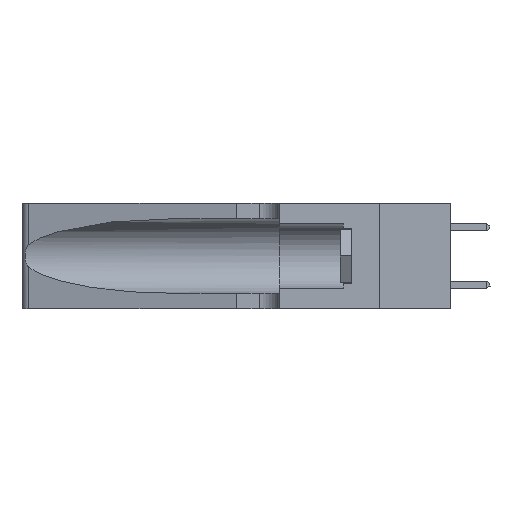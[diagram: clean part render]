
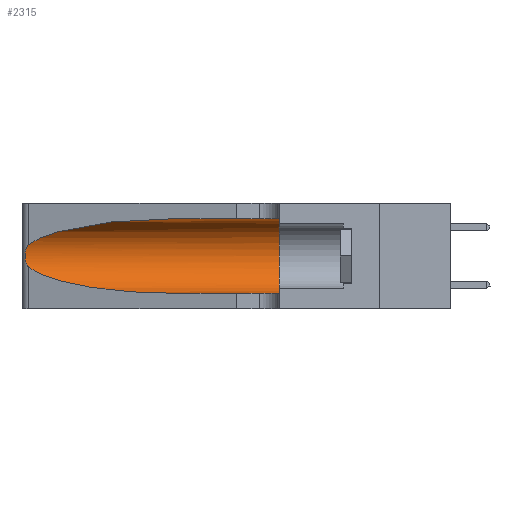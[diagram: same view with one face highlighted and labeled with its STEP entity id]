
A CAD part, left-side view. The second image highlights one B-rep face of the part: STEP entity #2315.
In plain terms, the highlighted cylindrical face has radius 3.308 mm (diameter 6.617 mm), a partial arc.
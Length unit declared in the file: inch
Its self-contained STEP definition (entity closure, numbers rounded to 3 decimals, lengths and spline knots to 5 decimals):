
#126 = CARTESIAN_POINT ( 'NONE',  ( 0.26018, 1.23835, 0.19895 ) ) ;
#447 = EDGE_CURVE ( 'NONE', #9253, #2792, #9507, .T. ) ;
#688 = CARTESIAN_POINT ( 'NONE',  ( 0.25487, 1.22718, 0.22369 ) ) ;
#937 =( BOUNDED_CURVE ( )  B_SPLINE_CURVE ( 3, ( #8725, #13086, #7332, #17427 ),
 .UNSPECIFIED., .F., .T. ) 
 B_SPLINE_CURVE_WITH_KNOTS ( ( 4, 4 ),
 ( 3.44316, 4.71239 ),
 .UNSPECIFIED. ) 
 CURVE ( )  GEOMETRIC_REPRESENTATION_ITEM ( )  RATIONAL_B_SPLINE_CURVE ( ( 1., 0.87, 0.87, 1. ) ) 
 REPRESENTATION_ITEM ( '' )  );
#1132 = EDGE_CURVE ( 'NONE', #12145, #8710, #11768, .T. ) ;
#1556 = DIRECTION ( 'NONE',  ( 0., -1., 0. ) ) ;
#1603 = CARTESIAN_POINT ( 'NONE',  ( 0.26075, 1.23896, 0.178 ) ) ;
#2315 = ADVANCED_FACE ( 'NONE', ( #3264 ), #13948, .F. ) ;
#2553 = VECTOR ( 'NONE', #12333, 39.37008 ) ;
#2683 = AXIS2_PLACEMENT_3D ( 'NONE', #3656, #12179, #5624 ) ;
#2792 = VERTEX_POINT ( 'NONE', #5924 ) ;
#3127 = CARTESIAN_POINT ( 'NONE',  ( 0.25856, 1.23593, 0.16098 ) ) ;
#3264 = FACE_OUTER_BOUND ( 'NONE', #5258, .T. ) ;
#3307 = EDGE_CURVE ( 'NONE', #7246, #2792, #6495, .T. ) ;
#3656 = CARTESIAN_POINT ( 'NONE',  ( 0.1305, 0.35, 0.185 ) ) ;
#4102 = ORIENTED_EDGE ( 'NONE', *, *, #3307, .T. ) ;
#4619 = CARTESIAN_POINT ( 'NONE',  ( 0.25639, 1.23186, 0.15144 ) ) ;
#4813 = DIRECTION ( 'NONE',  ( 0., -1., 0. ) ) ;
#5023 = CARTESIAN_POINT ( 'NONE',  ( 0.1305, 0.35, 0.31525 ) ) ;
#5258 = EDGE_LOOP ( 'NONE', ( #7559, #9914, #7156, #4102, #18725, #17137 ) ) ;
#5624 = DIRECTION ( 'NONE',  ( 0., 0., 1. ) ) ;
#5688 = AXIS2_PLACEMENT_3D ( 'NONE', #9655, #4813, #15910 ) ;
#5924 = CARTESIAN_POINT ( 'NONE',  ( 0.1305, 0.35, 0.05475 ) ) ;
#6111 = CARTESIAN_POINT ( 'NONE',  ( 0.25487, 1.22718, 0.14631 ) ) ;
#6495 = LINE ( 'NONE', #6636, #2553 ) ;
#6636 = CARTESIAN_POINT ( 'NONE',  ( 0.1305, 1.61858, 0.05475 ) ) ;
#6849 = VERTEX_POINT ( 'NONE', #12609 ) ;
#7074 = EDGE_CURVE ( 'NONE', #6849, #7246, #937, .T. ) ;
#7111 = CARTESIAN_POINT ( 'NONE',  ( 0.1305, 0.72297, 0.31525 ) ) ;
#7156 = ORIENTED_EDGE ( 'NONE', *, *, #7074, .T. ) ;
#7246 = VERTEX_POINT ( 'NONE', #10557 ) ;
#7332 = CARTESIAN_POINT ( 'NONE',  ( 0.18966, 0.96281, 0.05475 ) ) ;
#7487 = CARTESIAN_POINT ( 'NONE',  ( 0.25639, 1.23184, 0.21858 ) ) ;
#7559 = ORIENTED_EDGE ( 'NONE', *, *, #1132, .T. ) ;
#8710 = VERTEX_POINT ( 'NONE', #18006 ) ;
#8725 = CARTESIAN_POINT ( 'NONE',  ( 0.25487, 1.22718, 0.14631 ) ) ;
#8951 = CARTESIAN_POINT ( 'NONE',  ( 0.25854, 1.2359, 0.20912 ) ) ;
#9079 = VECTOR ( 'NONE', #1556, 39.37008 ) ;
#9253 = VERTEX_POINT ( 'NONE', #5023 ) ;
#9507 = CIRCLE ( 'NONE', #2683, 0.13025 ) ;
#9539 = EDGE_CURVE ( 'NONE', #12145, #9253, #16750, .T. ) ;
#9655 = CARTESIAN_POINT ( 'NONE',  ( 0.1305, 1.61858, 0.185 ) ) ;
#9914 = ORIENTED_EDGE ( 'NONE', *, *, #10138, .T. ) ;
#10138 = EDGE_CURVE ( 'NONE', #8710, #6849, #11512, .T. ) ;
#10402 = CARTESIAN_POINT ( 'NONE',  ( 0.26075, 1.23896, 0.19203 ) ) ;
#10557 = CARTESIAN_POINT ( 'NONE',  ( 0.1305, 0.72297, 0.05475 ) ) ;
#11512 = B_SPLINE_CURVE_WITH_KNOTS ( 'NONE', 3,
 ( #14697, #16137, #7487, #17583, #8951, #126, #10402, #1603, #11870, #3127, #13300, #4619, #14762, #6111 ),
 .UNSPECIFIED., .F., .F.,
 ( 4, 2, 2, 2, 2, 2, 4 ),
 ( 0., 0.00027, 0.00053, 0.00107, 0.0016, 0.00187, 0.00214 ),
 .UNSPECIFIED. ) ;
#11768 =( BOUNDED_CURVE ( )  B_SPLINE_CURVE ( 3, ( #7111, #17406, #16472, #688 ),
 .UNSPECIFIED., .F., .F. ) 
 B_SPLINE_CURVE_WITH_KNOTS ( ( 4, 4 ),
 ( 1.5708, 2.84003 ),
 .UNSPECIFIED. ) 
 CURVE ( )  GEOMETRIC_REPRESENTATION_ITEM ( )  RATIONAL_B_SPLINE_CURVE ( ( 1., 0.87, 0.87, 1. ) ) 
 REPRESENTATION_ITEM ( '' )  );
#11870 = CARTESIAN_POINT ( 'NONE',  ( 0.26017, 1.23833, 0.17102 ) ) ;
#12145 = VERTEX_POINT ( 'NONE', #13367 ) ;
#12179 = DIRECTION ( 'NONE',  ( 0., 1., 0. ) ) ;
#12333 = DIRECTION ( 'NONE',  ( 0., -1., 0. ) ) ;
#12609 = CARTESIAN_POINT ( 'NONE',  ( 0.25487, 1.22718, 0.14631 ) ) ;
#13086 = CARTESIAN_POINT ( 'NONE',  ( 0.2373, 1.15595, 0.08982 ) ) ;
#13300 = CARTESIAN_POINT ( 'NONE',  ( 0.25789, 1.23486, 0.15765 ) ) ;
#13367 = CARTESIAN_POINT ( 'NONE',  ( 0.1305, 0.72297, 0.31525 ) ) ;
#13948 = CYLINDRICAL_SURFACE ( 'NONE', #5688, 0.13025 ) ;
#14697 = CARTESIAN_POINT ( 'NONE',  ( 0.25487, 1.22718, 0.22369 ) ) ;
#14762 = CARTESIAN_POINT ( 'NONE',  ( 0.25555, 1.22993, 0.14849 ) ) ;
#15910 = DIRECTION ( 'NONE',  ( 0., 0., -1. ) ) ;
#16137 = CARTESIAN_POINT ( 'NONE',  ( 0.25555, 1.22994, 0.2215 ) ) ;
#16472 = CARTESIAN_POINT ( 'NONE',  ( 0.2373, 1.15595, 0.28018 ) ) ;
#16750 = LINE ( 'NONE', #17277, #9079 ) ;
#17137 = ORIENTED_EDGE ( 'NONE', *, *, #9539, .F. ) ;
#17277 = CARTESIAN_POINT ( 'NONE',  ( 0.1305, 1.61858, 0.31525 ) ) ;
#17406 = CARTESIAN_POINT ( 'NONE',  ( 0.18966, 0.96281, 0.31525 ) ) ;
#17427 = CARTESIAN_POINT ( 'NONE',  ( 0.1305, 0.72297, 0.05475 ) ) ;
#17583 = CARTESIAN_POINT ( 'NONE',  ( 0.25787, 1.23484, 0.2124 ) ) ;
#18006 = CARTESIAN_POINT ( 'NONE',  ( 0.25487, 1.22718, 0.22369 ) ) ;
#18725 = ORIENTED_EDGE ( 'NONE', *, *, #447, .F. ) ;
